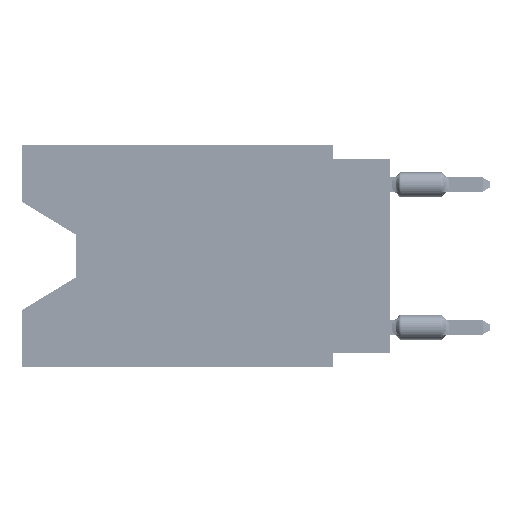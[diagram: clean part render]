
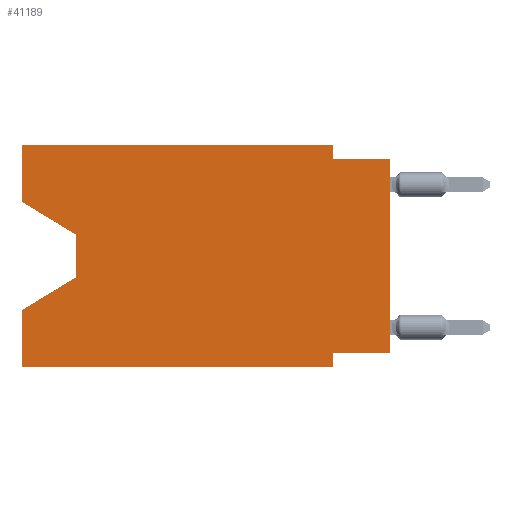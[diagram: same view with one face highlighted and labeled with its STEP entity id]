
A CAD part, left-side view. The second image highlights one B-rep face of the part: STEP entity #41189.
In plain terms, the highlighted planar face has unit normal (-1, 0, 0).
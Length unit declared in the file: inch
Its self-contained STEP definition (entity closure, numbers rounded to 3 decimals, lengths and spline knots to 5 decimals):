
#119 = CARTESIAN_POINT ( 'NONE',  ( 0., 0.1, -0.365 ) ) ;
#361 = CARTESIAN_POINT ( 'NONE',  ( 0., 0.645, -0.28975 ) ) ;
#788 = CARTESIAN_POINT ( 'NONE',  ( 0., 0.645, -0.10025 ) ) ;
#1942 = CARTESIAN_POINT ( 'NONE',  ( 0., 0.55, -0.158 ) ) ;
#2287 = ORIENTED_EDGE ( 'NONE', *, *, #63301, .F. ) ;
#4010 = VECTOR ( 'NONE', #23599, 39.37008 ) ;
#4343 = LINE ( 'NONE', #5969, #66650 ) ;
#4929 = VECTOR ( 'NONE', #35982, 39.37008 ) ;
#5969 = CARTESIAN_POINT ( 'NONE',  ( 0., 0.645, 0. ) ) ;
#6973 = CARTESIAN_POINT ( 'NONE',  ( 0., 0., 0. ) ) ;
#7248 = VECTOR ( 'NONE', #43144, 39.37008 ) ;
#8040 = FACE_OUTER_BOUND ( 'NONE', #53847, .T. ) ;
#10004 = EDGE_CURVE ( 'NONE', #54733, #39632, #63720, .T. ) ;
#10467 = ORIENTED_EDGE ( 'NONE', *, *, #47257, .T. ) ;
#10720 = CARTESIAN_POINT ( 'NONE',  ( 0., 0.645, 0. ) ) ;
#10772 = LINE ( 'NONE', #49682, #4010 ) ;
#12736 = VECTOR ( 'NONE', #15943, 39.37008 ) ;
#12827 = EDGE_CURVE ( 'NONE', #63374, #58020, #10772, .T. ) ;
#13840 = ORIENTED_EDGE ( 'NONE', *, *, #12827, .F. ) ;
#14270 = DIRECTION ( 'NONE',  ( 1., 0., 0. ) ) ;
#15068 = PLANE ( 'NONE',  #19596 ) ;
#15593 = CARTESIAN_POINT ( 'NONE',  ( 0., 0.1, -0.025 ) ) ;
#15943 = DIRECTION ( 'NONE',  ( 0., 0., 1. ) ) ;
#18313 = VERTEX_POINT ( 'NONE', #361 ) ;
#18371 = VECTOR ( 'NONE', #37407, 39.37008 ) ;
#18662 = VERTEX_POINT ( 'NONE', #59549 ) ;
#18672 = ORIENTED_EDGE ( 'NONE', *, *, #80522, .T. ) ;
#18966 = CARTESIAN_POINT ( 'NONE',  ( 0., 0.1, 0. ) ) ;
#19504 = EDGE_CURVE ( 'NONE', #80162, #21593, #52496, .T. ) ;
#19596 = AXIS2_PLACEMENT_3D ( 'NONE', #58986, #14270, #65194 ) ;
#21593 = VERTEX_POINT ( 'NONE', #61163 ) ;
#23599 = DIRECTION ( 'NONE',  ( 0., 0., -1. ) ) ;
#25728 = CARTESIAN_POINT ( 'NONE',  ( 0., 0.645, -0.39 ) ) ;
#26738 = VECTOR ( 'NONE', #39659, 39.37008 ) ;
#27745 = CARTESIAN_POINT ( 'NONE',  ( 0., 0., -0.025 ) ) ;
#28152 = LINE ( 'NONE', #27745, #55621 ) ;
#28778 = LINE ( 'NONE', #48660, #12736 ) ;
#29891 = EDGE_CURVE ( 'NONE', #18662, #80162, #45945, .T. ) ;
#33441 = VECTOR ( 'NONE', #80507, 39.37008 ) ;
#35815 = LINE ( 'NONE', #60244, #33441 ) ;
#35982 = DIRECTION ( 'NONE',  ( 0., -1., 0. ) ) ;
#37191 = CARTESIAN_POINT ( 'NONE',  ( 0., 0., -0.365 ) ) ;
#37407 = DIRECTION ( 'NONE',  ( 0., 0., -1. ) ) ;
#39632 = VERTEX_POINT ( 'NONE', #46251 ) ;
#39659 = DIRECTION ( 'NONE',  ( 0., 0., -1. ) ) ;
#41189 = ADVANCED_FACE ( 'NONE', ( #8040 ), #15068, .F. ) ;
#42798 = VECTOR ( 'NONE', #57519, 39.37008 ) ;
#43144 = DIRECTION ( 'NONE',  ( 0., 0.855, -0.519 ) ) ;
#43269 = DIRECTION ( 'NONE',  ( 0., 0., 1. ) ) ;
#43547 = CARTESIAN_POINT ( 'NONE',  ( 0., 0.55, -0.232 ) ) ;
#43810 = VERTEX_POINT ( 'NONE', #25728 ) ;
#44598 = EDGE_CURVE ( 'NONE', #43810, #18313, #4343, .T. ) ;
#44611 = ORIENTED_EDGE ( 'NONE', *, *, #19504, .T. ) ;
#45945 = LINE ( 'NONE', #788, #73551 ) ;
#46251 = CARTESIAN_POINT ( 'NONE',  ( 0., 0., -0.025 ) ) ;
#47257 = EDGE_CURVE ( 'NONE', #21593, #18313, #49355, .T. ) ;
#47710 = ORIENTED_EDGE ( 'NONE', *, *, #29891, .T. ) ;
#48660 = CARTESIAN_POINT ( 'NONE',  ( 0., 0.645, 0. ) ) ;
#49355 = LINE ( 'NONE', #43547, #7248 ) ;
#49419 = VERTEX_POINT ( 'NONE', #52449 ) ;
#49682 = CARTESIAN_POINT ( 'NONE',  ( 0., 0.1, 0. ) ) ;
#50791 = CARTESIAN_POINT ( 'NONE',  ( 0., 0.55, -0.158 ) ) ;
#52449 = CARTESIAN_POINT ( 'NONE',  ( 0., 0.1, -0.39 ) ) ;
#52496 = LINE ( 'NONE', #1942, #26738 ) ;
#53678 = ORIENTED_EDGE ( 'NONE', *, *, #61271, .F. ) ;
#53847 = EDGE_LOOP ( 'NONE', ( #47710, #44611, #10467, #71881, #18672, #67216, #81510, #78297, #63910, #13840, #2287, #53678 ) ) ;
#54412 = LINE ( 'NONE', #67645, #18371 ) ;
#54733 = VERTEX_POINT ( 'NONE', #37191 ) ;
#55621 = VECTOR ( 'NONE', #78239, 39.37008 ) ;
#57519 = DIRECTION ( 'NONE',  ( 0., 0., 1. ) ) ;
#58020 = VERTEX_POINT ( 'NONE', #15593 ) ;
#58525 = VERTEX_POINT ( 'NONE', #65224 ) ;
#58986 = CARTESIAN_POINT ( 'NONE',  ( 0., 0.645, 0. ) ) ;
#59549 = CARTESIAN_POINT ( 'NONE',  ( 0., 0.645, -0.10025 ) ) ;
#60079 = EDGE_CURVE ( 'NONE', #54733, #63029, #74581, .T. ) ;
#60244 = CARTESIAN_POINT ( 'NONE',  ( 0., 0.645, -0.39 ) ) ;
#61163 = CARTESIAN_POINT ( 'NONE',  ( 0., 0.55, -0.232 ) ) ;
#61271 = EDGE_CURVE ( 'NONE', #18662, #58525, #28778, .T. ) ;
#63029 = VERTEX_POINT ( 'NONE', #119 ) ;
#63301 = EDGE_CURVE ( 'NONE', #58525, #63374, #67446, .T. ) ;
#63374 = VERTEX_POINT ( 'NONE', #18966 ) ;
#63720 = LINE ( 'NONE', #6973, #42798 ) ;
#63910 = ORIENTED_EDGE ( 'NONE', *, *, #77707, .F. ) ;
#64570 = DIRECTION ( 'NONE',  ( 0., -0.855, -0.519 ) ) ;
#65194 = DIRECTION ( 'NONE',  ( 0., 0., -1. ) ) ;
#65224 = CARTESIAN_POINT ( 'NONE',  ( 0., 0.645, 0. ) ) ;
#66650 = VECTOR ( 'NONE', #43269, 39.37008 ) ;
#66997 = VECTOR ( 'NONE', #81210, 39.37008 ) ;
#67216 = ORIENTED_EDGE ( 'NONE', *, *, #75827, .F. ) ;
#67446 = LINE ( 'NONE', #10720, #4929 ) ;
#67645 = CARTESIAN_POINT ( 'NONE',  ( 0., 0.1, -0.39 ) ) ;
#71881 = ORIENTED_EDGE ( 'NONE', *, *, #44598, .F. ) ;
#73551 = VECTOR ( 'NONE', #64570, 39.37008 ) ;
#74581 = LINE ( 'NONE', #79977, #66997 ) ;
#75827 = EDGE_CURVE ( 'NONE', #63029, #49419, #54412, .T. ) ;
#77707 = EDGE_CURVE ( 'NONE', #58020, #39632, #28152, .T. ) ;
#78239 = DIRECTION ( 'NONE',  ( 0., -1., 0. ) ) ;
#78297 = ORIENTED_EDGE ( 'NONE', *, *, #10004, .T. ) ;
#79977 = CARTESIAN_POINT ( 'NONE',  ( 0., 0., -0.365 ) ) ;
#80162 = VERTEX_POINT ( 'NONE', #50791 ) ;
#80507 = DIRECTION ( 'NONE',  ( 0., -1., 0. ) ) ;
#80522 = EDGE_CURVE ( 'NONE', #43810, #49419, #35815, .T. ) ;
#81210 = DIRECTION ( 'NONE',  ( 0., 1., 0. ) ) ;
#81510 = ORIENTED_EDGE ( 'NONE', *, *, #60079, .F. ) ;
